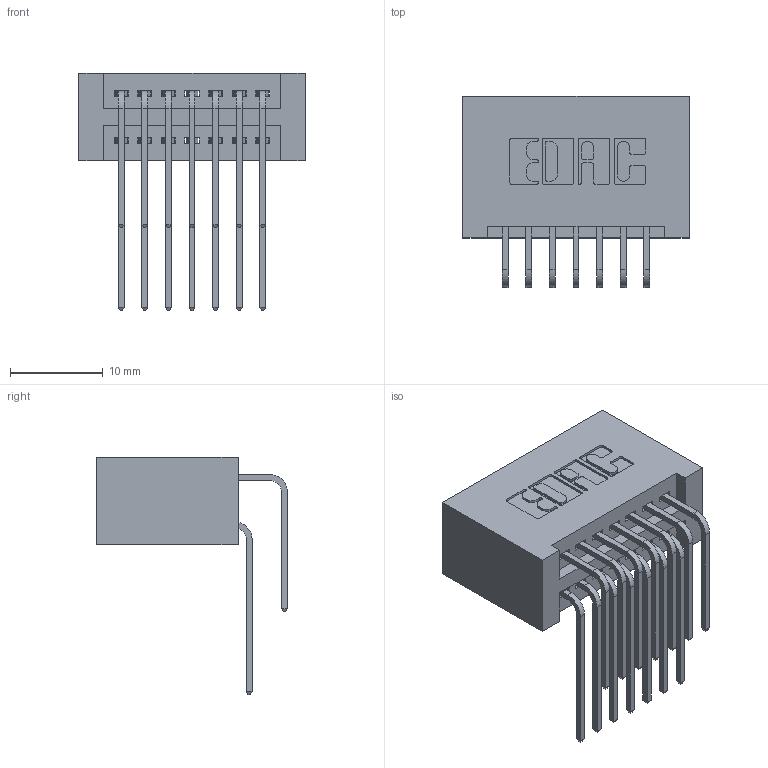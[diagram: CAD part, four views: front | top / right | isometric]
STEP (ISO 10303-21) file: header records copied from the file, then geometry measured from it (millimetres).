
FILE_DESCRIPTION (( 'STEP AP203' ), '1' );
FILE_NAME ('395-014-559-201.STEP', '2019-10-15T16:57:03', ( '' ), ( '' ), 'SwSTEP 2.0', 'SolidWorks 2016', '' );
FILE_SCHEMA (( 'CONFIG_CONTROL_DESIGN' ));
Length unit declared in the file: inch
Products named in the file (4): 345 Part_No Mounting Lugs; 345-292-001_558 559 Tail - 1; 345-292-001_559 Tail - 2; 395-014-559-201
Assembly tree (15 placements, depth 2):
  395-014-559-201
    345 Part_No Mounting Lugs
    345-292-001_558 559 Tail - 1  x7
    345-292-001_559 Tail - 2  x7
Bounding box: 24.38 x 20.56 x 25.53 mm (x, y, z)
Volume: 2740.5 mm3; surface area: 4056 mm2
Topology: 15 solids, 15 shells, 846 faces, 2487 edges, 1638 vertices
Faces by surface type: plane 566, cylinder 280
Entity records: 11579 total; most frequent: CARTESIAN_POINT 2019, ORIENTED_EDGE 1902, DIRECTION 1791, EDGE_CURVE 951, VECTOR 759, LINE 759, VERTEX_POINT 630, AXIS2_PLACEMENT_3D 516
